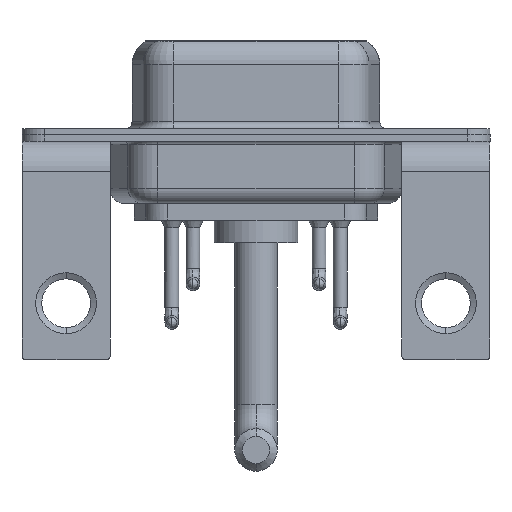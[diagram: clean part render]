
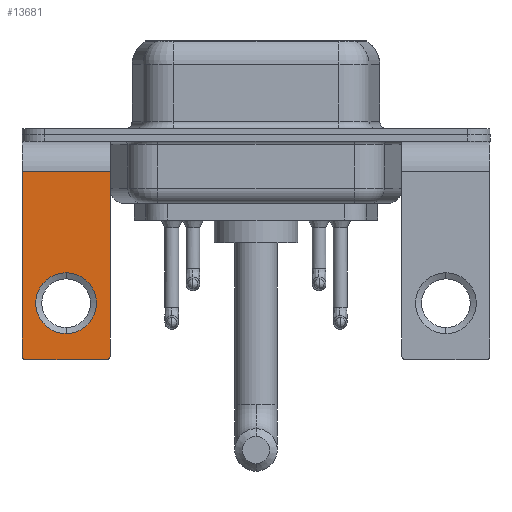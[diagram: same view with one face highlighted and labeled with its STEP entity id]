
A CAD part, front view. The second image highlights one B-rep face of the part: STEP entity #13681.
In plain terms, the highlighted planar face has unit normal (0, -1, 0).
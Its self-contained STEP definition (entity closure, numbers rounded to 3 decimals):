
#297 = VERTEX_POINT ( 'NONE', #1072 ) ;
#354 = FACE_BOUND ( 'NONE', #9040, .T. ) ;
#572 = CARTESIAN_POINT ( 'NONE',  ( 0., -6.25, -13.07 ) ) ;
#1072 = CARTESIAN_POINT ( 'NONE',  ( -2.9, -6.25, -14.55 ) ) ;
#1316 = CARTESIAN_POINT ( 'NONE',  ( 2.9, -6.25, -2.4 ) ) ;
#1606 = AXIS2_PLACEMENT_3D ( 'NONE', #5451, #9187, #9524 ) ;
#2128 = ORIENTED_EDGE ( 'NONE', *, *, #5842, .T. ) ;
#2186 = CARTESIAN_POINT ( 'NONE',  ( -2.9, -6.25, -2.4 ) ) ;
#2703 = ORIENTED_EDGE ( 'NONE', *, *, #6546, .T. ) ;
#2744 = DIRECTION ( 'NONE',  ( 0., 0., -1. ) ) ;
#2906 = LINE ( 'NONE', #8274, #8491 ) ;
#2931 = EDGE_CURVE ( 'NONE', #11310, #7268, #8472, .T. ) ;
#3107 = DIRECTION ( 'NONE',  ( 0., -1., 0. ) ) ;
#3185 = DIRECTION ( 'NONE',  ( 0., 0., 1. ) ) ;
#3215 = VERTEX_POINT ( 'NONE', #14671 ) ;
#3268 = PLANE ( 'NONE',  #7842 ) ;
#3662 = VERTEX_POINT ( 'NONE', #572 ) ;
#3666 = LINE ( 'NONE', #2186, #7783 ) ;
#3750 = EDGE_CURVE ( 'NONE', #297, #7268, #15373, .T. ) ;
#4269 = ORIENTED_EDGE ( 'NONE', *, *, #2931, .F. ) ;
#4483 = EDGE_CURVE ( 'NONE', #5103, #9495, #2906, .T. ) ;
#5091 = VERTEX_POINT ( 'NONE', #16443 ) ;
#5103 = VERTEX_POINT ( 'NONE', #8611 ) ;
#5451 = CARTESIAN_POINT ( 'NONE',  ( 0., -6.25, -11.07 ) ) ;
#5787 = CARTESIAN_POINT ( 'NONE',  ( 2.9, -6.25, -2.4 ) ) ;
#5842 = EDGE_CURVE ( 'NONE', #5103, #3215, #17019, .T. ) ;
#5920 = AXIS2_PLACEMENT_3D ( 'NONE', #8200, #3107, #6998 ) ;
#6418 = CARTESIAN_POINT ( 'NONE',  ( -2.65, -6.25, -14.55 ) ) ;
#6546 = EDGE_CURVE ( 'NONE', #3662, #5091, #7125, .T. ) ;
#6998 = DIRECTION ( 'NONE',  ( 0., 0., 1. ) ) ;
#7125 = CIRCLE ( 'NONE', #1606, 2. ) ;
#7268 = VERTEX_POINT ( 'NONE', #11411 ) ;
#7625 = DIRECTION ( 'NONE',  ( 0., 0., -1. ) ) ;
#7783 = VECTOR ( 'NONE', #7625, 1000. ) ;
#7842 = AXIS2_PLACEMENT_3D ( 'NONE', #5787, #9693, #3185 ) ;
#7896 = CARTESIAN_POINT ( 'NONE',  ( 2.9, -6.25, -14.55 ) ) ;
#8200 = CARTESIAN_POINT ( 'NONE',  ( 2.65, -6.25, -14.55 ) ) ;
#8274 = CARTESIAN_POINT ( 'NONE',  ( 2.9, -6.25, -2.4 ) ) ;
#8393 = ORIENTED_EDGE ( 'NONE', *, *, #10536, .T. ) ;
#8472 = LINE ( 'NONE', #13744, #12617 ) ;
#8491 = VECTOR ( 'NONE', #2744, 1000. ) ;
#8611 = CARTESIAN_POINT ( 'NONE',  ( 2.9, -6.25, -2.4 ) ) ;
#8718 = ORIENTED_EDGE ( 'NONE', *, *, #4483, .F. ) ;
#8868 = AXIS2_PLACEMENT_3D ( 'NONE', #11444, #13928, #15376 ) ;
#9040 = EDGE_LOOP ( 'NONE', ( #2703, #8393 ) ) ;
#9187 = DIRECTION ( 'NONE',  ( 0., 1., 0. ) ) ;
#9272 = DIRECTION ( 'NONE',  ( -1., 0., 0. ) ) ;
#9355 = DIRECTION ( 'NONE',  ( 0., -1., 0. ) ) ;
#9495 = VERTEX_POINT ( 'NONE', #7896 ) ;
#9524 = DIRECTION ( 'NONE',  ( 0., 0., 1. ) ) ;
#9693 = DIRECTION ( 'NONE',  ( 0., 1., 0. ) ) ;
#9982 = CIRCLE ( 'NONE', #8868, 2. ) ;
#10299 = DIRECTION ( 'NONE',  ( -1., 0., 0. ) ) ;
#10536 = EDGE_CURVE ( 'NONE', #5091, #3662, #9982, .T. ) ;
#10926 = ORIENTED_EDGE ( 'NONE', *, *, #13563, .T. ) ;
#10980 = AXIS2_PLACEMENT_3D ( 'NONE', #6418, #9355, #12989 ) ;
#11168 = FACE_OUTER_BOUND ( 'NONE', #16641, .T. ) ;
#11183 = CIRCLE ( 'NONE', #5920, 0.25 ) ;
#11310 = VERTEX_POINT ( 'NONE', #11672 ) ;
#11411 = CARTESIAN_POINT ( 'NONE',  ( -2.65, -6.25, -14.8 ) ) ;
#11444 = CARTESIAN_POINT ( 'NONE',  ( 0., -6.25, -11.07 ) ) ;
#11546 = EDGE_CURVE ( 'NONE', #3215, #297, #3666, .T. ) ;
#11672 = CARTESIAN_POINT ( 'NONE',  ( 2.65, -6.25, -14.8 ) ) ;
#12617 = VECTOR ( 'NONE', #10299, 1000. ) ;
#12651 = VECTOR ( 'NONE', #9272, 1000. ) ;
#12989 = DIRECTION ( 'NONE',  ( 0., 0., 1. ) ) ;
#13563 = EDGE_CURVE ( 'NONE', #11310, #9495, #11183, .T. ) ;
#13681 = ADVANCED_FACE ( 'NONE', ( #354, #11168 ), #3268, .F. ) ;
#13744 = CARTESIAN_POINT ( 'NONE',  ( 2.9, -6.25, -14.8 ) ) ;
#13928 = DIRECTION ( 'NONE',  ( 0., 1., 0. ) ) ;
#13940 = ORIENTED_EDGE ( 'NONE', *, *, #11546, .T. ) ;
#14671 = CARTESIAN_POINT ( 'NONE',  ( -2.9, -6.25, -2.4 ) ) ;
#15373 = CIRCLE ( 'NONE', #10980, 0.25 ) ;
#15376 = DIRECTION ( 'NONE',  ( 0., 0., 1. ) ) ;
#16101 = ORIENTED_EDGE ( 'NONE', *, *, #3750, .T. ) ;
#16443 = CARTESIAN_POINT ( 'NONE',  ( 0., -6.25, -9.07 ) ) ;
#16641 = EDGE_LOOP ( 'NONE', ( #13940, #16101, #4269, #10926, #8718, #2128 ) ) ;
#17019 = LINE ( 'NONE', #1316, #12651 ) ;
